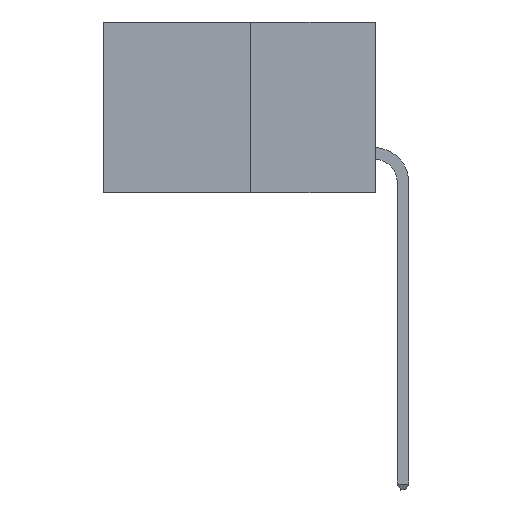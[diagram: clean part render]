
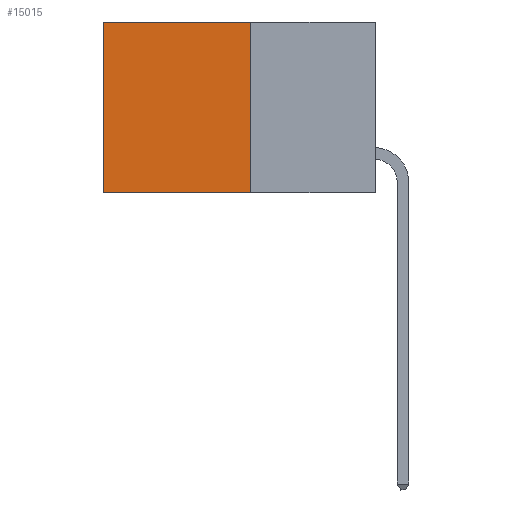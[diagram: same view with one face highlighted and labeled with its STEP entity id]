
A CAD part, left-side view. The second image highlights one B-rep face of the part: STEP entity #15015.
In plain terms, the highlighted planar face has unit normal (-1, 0, 0).
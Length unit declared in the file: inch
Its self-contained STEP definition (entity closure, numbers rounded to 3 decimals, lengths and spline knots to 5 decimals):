
#128 = VERTEX_POINT ( 'NONE', #10776 ) ;
#229 = CARTESIAN_POINT ( 'NONE',  ( 0.277, 0.27, 0. ) ) ;
#1749 = DIRECTION ( 'NONE',  ( 0., 1., 0. ) ) ;
#1858 = CARTESIAN_POINT ( 'NONE',  ( 0.277, 0.27, -0.37 ) ) ;
#2735 = AXIS2_PLACEMENT_3D ( 'NONE', #11871, #6730, #18754 ) ;
#3396 = VECTOR ( 'NONE', #1749, 39.37008 ) ;
#3799 = VECTOR ( 'NONE', #8866, 39.37008 ) ;
#3937 = VERTEX_POINT ( 'NONE', #15765 ) ;
#4366 = LINE ( 'NONE', #7030, #3799 ) ;
#4540 = VERTEX_POINT ( 'NONE', #6976 ) ;
#4873 = DIRECTION ( 'NONE',  ( 0., 1., 0. ) ) ;
#4980 = ORIENTED_EDGE ( 'NONE', *, *, #20026, .T. ) ;
#5009 = FACE_OUTER_BOUND ( 'NONE', #13506, .T. ) ;
#5012 = PLANE ( 'NONE',  #2735 ) ;
#5520 = DIRECTION ( 'NONE',  ( 0., 0., -1. ) ) ;
#6180 = EDGE_CURVE ( 'NONE', #4540, #128, #7990, .T. ) ;
#6730 = DIRECTION ( 'NONE',  ( 1., 0., 0. ) ) ;
#6976 = CARTESIAN_POINT ( 'NONE',  ( 0.277, 0.27, -0.37 ) ) ;
#7030 = CARTESIAN_POINT ( 'NONE',  ( 0.277, 0.27, -0.37 ) ) ;
#7990 = LINE ( 'NONE', #1858, #3396 ) ;
#8145 = VECTOR ( 'NONE', #5520, 39.37008 ) ;
#8649 = VECTOR ( 'NONE', #4873, 39.37008 ) ;
#8762 = ORIENTED_EDGE ( 'NONE', *, *, #6180, .F. ) ;
#8866 = DIRECTION ( 'NONE',  ( 0., 0., -1. ) ) ;
#9197 = EDGE_CURVE ( 'NONE', #15740, #4540, #4366, .T. ) ;
#10776 = CARTESIAN_POINT ( 'NONE',  ( 0.277, 0.59, -0.37 ) ) ;
#11871 = CARTESIAN_POINT ( 'NONE',  ( 0.277, 0.27, -0.37 ) ) ;
#13245 = LINE ( 'NONE', #16894, #8649 ) ;
#13506 = EDGE_LOOP ( 'NONE', ( #20240, #8762, #22070, #4980 ) ) ;
#14128 = CARTESIAN_POINT ( 'NONE',  ( 0.277, 0.59, -0.37 ) ) ;
#15015 = ADVANCED_FACE ( 'NONE', ( #5009 ), #5012, .F. ) ;
#15740 = VERTEX_POINT ( 'NONE', #229 ) ;
#15765 = CARTESIAN_POINT ( 'NONE',  ( 0.277, 0.59, 0. ) ) ;
#16751 = LINE ( 'NONE', #14128, #8145 ) ;
#16894 = CARTESIAN_POINT ( 'NONE',  ( 0.277, 0.27, 0. ) ) ;
#18754 = DIRECTION ( 'NONE',  ( 0., 0., -1. ) ) ;
#18819 = EDGE_CURVE ( 'NONE', #3937, #128, #16751, .T. ) ;
#20026 = EDGE_CURVE ( 'NONE', #15740, #3937, #13245, .T. ) ;
#20240 = ORIENTED_EDGE ( 'NONE', *, *, #18819, .T. ) ;
#22070 = ORIENTED_EDGE ( 'NONE', *, *, #9197, .F. ) ;
